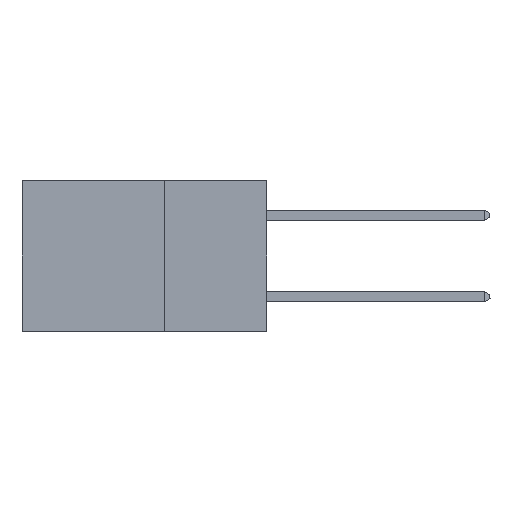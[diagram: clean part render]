
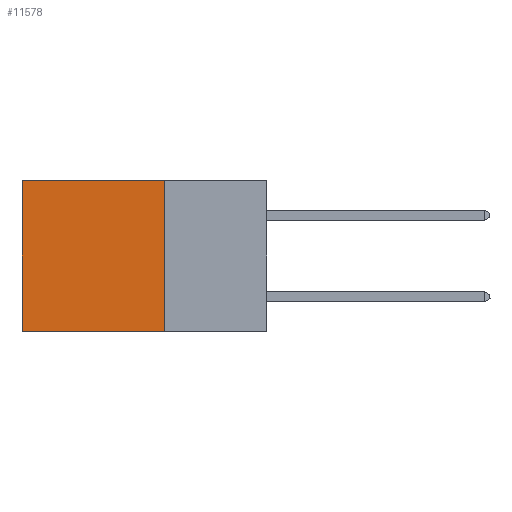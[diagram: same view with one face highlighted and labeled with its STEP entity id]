
A CAD part, left-side view. The second image highlights one B-rep face of the part: STEP entity #11578.
In plain terms, the highlighted planar face has unit normal (-1, 0, 0).
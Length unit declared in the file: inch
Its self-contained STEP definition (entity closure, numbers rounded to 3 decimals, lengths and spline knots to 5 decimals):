
#1358 = EDGE_CURVE ( 'NONE', #14332, #12378, #32916, .T. ) ;
#3400 = ORIENTED_EDGE ( 'NONE', *, *, #35649, .F. ) ;
#4058 = ORIENTED_EDGE ( 'NONE', *, *, #1358, .T. ) ;
#5147 = EDGE_CURVE ( 'NONE', #22671, #7981, #36513, .T. ) ;
#5261 = DIRECTION ( 'NONE',  ( 0., 0., -1. ) ) ;
#6005 = AXIS2_PLACEMENT_3D ( 'NONE', #25246, #19324, #5261 ) ;
#7981 = VERTEX_POINT ( 'NONE', #30920 ) ;
#9627 = LINE ( 'NONE', #21361, #27232 ) ;
#9642 = DIRECTION ( 'NONE',  ( 0., 0., -1. ) ) ;
#10169 = EDGE_LOOP ( 'NONE', ( #4058, #3400, #30462, #19207 ) ) ;
#10185 = DIRECTION ( 'NONE',  ( 0., 0., -1. ) ) ;
#11334 = VECTOR ( 'NONE', #10185, 39.37008 ) ;
#11578 = ADVANCED_FACE ( 'NONE', ( #28531 ), #14093, .F. ) ;
#12378 = VERTEX_POINT ( 'NONE', #25653 ) ;
#12573 = CARTESIAN_POINT ( 'NONE',  ( 0.2875, 0.25, 0. ) ) ;
#13538 = VECTOR ( 'NONE', #9642, 39.37008 ) ;
#14093 = PLANE ( 'NONE',  #6005 ) ;
#14332 = VERTEX_POINT ( 'NONE', #18312 ) ;
#15790 = DIRECTION ( 'NONE',  ( 0., 1., 0. ) ) ;
#16019 = CARTESIAN_POINT ( 'NONE',  ( 0.2875, 0.25, 0. ) ) ;
#18312 = CARTESIAN_POINT ( 'NONE',  ( 0.2875, 0.6, 0. ) ) ;
#18921 = LINE ( 'NONE', #12573, #32115 ) ;
#19207 = ORIENTED_EDGE ( 'NONE', *, *, #35226, .T. ) ;
#19324 = DIRECTION ( 'NONE',  ( 1., 0., 0. ) ) ;
#21361 = CARTESIAN_POINT ( 'NONE',  ( 0.2875, 0.25, -0.37 ) ) ;
#22671 = VERTEX_POINT ( 'NONE', #16019 ) ;
#24291 = DIRECTION ( 'NONE',  ( 0., 1., 0. ) ) ;
#25246 = CARTESIAN_POINT ( 'NONE',  ( 0.2875, 0.25, 0. ) ) ;
#25653 = CARTESIAN_POINT ( 'NONE',  ( 0.2875, 0.6, -0.37 ) ) ;
#26902 = CARTESIAN_POINT ( 'NONE',  ( 0.2875, 0.25, 0. ) ) ;
#27232 = VECTOR ( 'NONE', #15790, 39.37008 ) ;
#28531 = FACE_OUTER_BOUND ( 'NONE', #10169, .T. ) ;
#30462 = ORIENTED_EDGE ( 'NONE', *, *, #5147, .F. ) ;
#30920 = CARTESIAN_POINT ( 'NONE',  ( 0.2875, 0.25, -0.37 ) ) ;
#32115 = VECTOR ( 'NONE', #24291, 39.37008 ) ;
#32916 = LINE ( 'NONE', #37772, #13538 ) ;
#35226 = EDGE_CURVE ( 'NONE', #22671, #14332, #18921, .T. ) ;
#35649 = EDGE_CURVE ( 'NONE', #7981, #12378, #9627, .T. ) ;
#36513 = LINE ( 'NONE', #26902, #11334 ) ;
#37772 = CARTESIAN_POINT ( 'NONE',  ( 0.2875, 0.6, 0. ) ) ;
